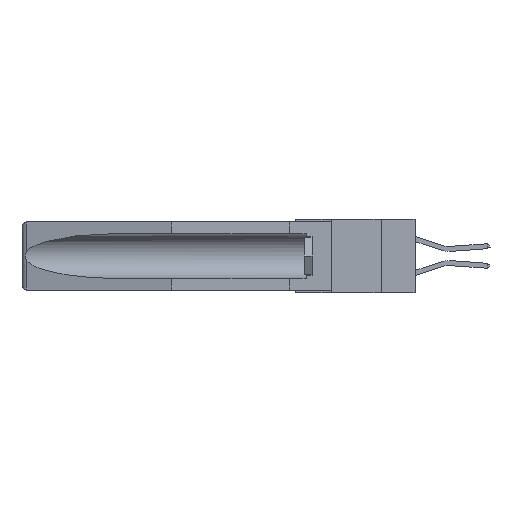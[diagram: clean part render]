
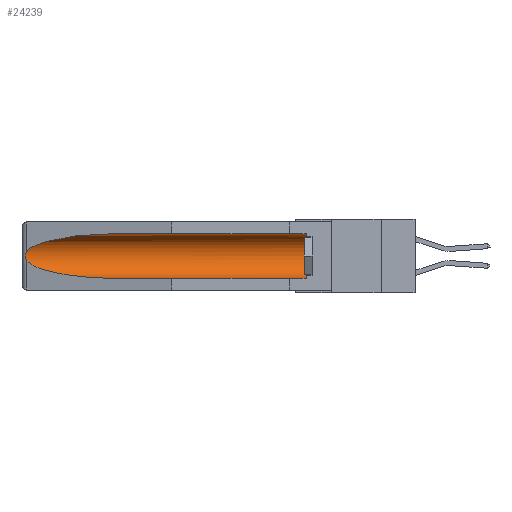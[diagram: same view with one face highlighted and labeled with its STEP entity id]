
A CAD part, left-side view. The second image highlights one B-rep face of the part: STEP entity #24239.
In plain terms, the highlighted cylindrical face has radius 2.857 mm (diameter 5.715 mm), a partial arc.
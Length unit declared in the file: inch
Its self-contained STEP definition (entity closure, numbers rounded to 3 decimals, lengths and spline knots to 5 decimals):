
#171 = CARTESIAN_POINT ( 'NONE',  ( 0.155, 1.07973, -0.284 ) ) ;
#558 = CARTESIAN_POINT ( 'NONE',  ( 0.25451, 1.48313, -0.09465 ) ) ;
#1365 = CARTESIAN_POINT ( 'NONE',  ( 0.26537, 1.52718, -0.19328 ) ) ;
#1795 = B_SPLINE_CURVE_WITH_KNOTS ( 'NONE', 3,
 ( #27884, #16819, #12589, #3488, #19022, #5691, #16997, #21360, #25749, #8009 ),
 .UNSPECIFIED., .F., .F.,
 ( 4, 2, 2, 2, 4 ),
 ( 0., 0.00029, 0.00058, 0.00087, 0.00117 ),
 .UNSPECIFIED. ) ;
#1805 = VERTEX_POINT ( 'NONE', #1365 ) ;
#3039 = EDGE_CURVE ( 'NONE', #3858, #21235, #5932, .T. ) ;
#3051 =( BOUNDED_CURVE ( )  B_SPLINE_CURVE ( 3, ( #9371, #20588, #558, #18332 ),
 .UNSPECIFIED., .F., .F. ) 
 B_SPLINE_CURVE_WITH_KNOTS ( ( 4, 4 ),
 ( 4.71239, 6.08839 ),
 .UNSPECIFIED. ) 
 CURVE ( )  GEOMETRIC_REPRESENTATION_ITEM ( )  RATIONAL_B_SPLINE_CURVE ( ( 1., 0.848, 0.848, 1. ) ) 
 REPRESENTATION_ITEM ( '' )  );
#3488 = CARTESIAN_POINT ( 'NONE',  ( 0.2673, 1.5327, -0.16383 ) ) ;
#3831 = VERTEX_POINT ( 'NONE', #23827 ) ;
#3858 = VERTEX_POINT ( 'NONE', #28498 ) ;
#5331 = DIRECTION ( 'NONE',  ( 0., 1., 0. ) ) ;
#5691 = CARTESIAN_POINT ( 'NONE',  ( 0.2675, 1.53308, -0.17534 ) ) ;
#5852 = VECTOR ( 'NONE', #23564, 39.37008 ) ;
#5932 = CIRCLE ( 'NONE', #6307, 0.1125 ) ;
#6307 = AXIS2_PLACEMENT_3D ( 'NONE', #20784, #16509, #18625 ) ;
#7411 = DIRECTION ( 'NONE',  ( 0., 1., 0. ) ) ;
#7586 = VECTOR ( 'NONE', #7411, 39.37008 ) ;
#8009 = CARTESIAN_POINT ( 'NONE',  ( 0.26537, 1.52718, -0.19328 ) ) ;
#8056 = CARTESIAN_POINT ( 'NONE',  ( 0.26537, 1.52718, -0.19328 ) ) ;
#8561 = ORIENTED_EDGE ( 'NONE', *, *, #3039, .T. ) ;
#9371 = CARTESIAN_POINT ( 'NONE',  ( 0.155, 1.07973, -0.059 ) ) ;
#9714 = LINE ( 'NONE', #23178, #5852 ) ;
#10353 = VERTEX_POINT ( 'NONE', #27807 ) ;
#11730 = CARTESIAN_POINT ( 'NONE',  ( 0.155, 0.126, -0.059 ) ) ;
#12170 = CARTESIAN_POINT ( 'NONE',  ( 0.155, -0.30754, -0.284 ) ) ;
#12542 = CARTESIAN_POINT ( 'NONE',  ( 0.21114, 1.30732, -0.284 ) ) ;
#12589 = CARTESIAN_POINT ( 'NONE',  ( 0.26654, 1.53092, -0.15636 ) ) ;
#13919 = AXIS2_PLACEMENT_3D ( 'NONE', #16935, #5331, #20921 ) ;
#14865 = EDGE_LOOP ( 'NONE', ( #19774, #23421, #25282, #19618, #8561, #22807 ) ) ;
#15461 = EDGE_CURVE ( 'NONE', #3831, #10353, #3051, .T. ) ;
#16509 = DIRECTION ( 'NONE',  ( 0., -1., 0. ) ) ;
#16819 = CARTESIAN_POINT ( 'NONE',  ( 0.26597, 1.52961, -0.15275 ) ) ;
#16935 = CARTESIAN_POINT ( 'NONE',  ( 0.155, -0.30754, -0.1715 ) ) ;
#16997 = CARTESIAN_POINT ( 'NONE',  ( 0.2673, 1.53269, -0.17917 ) ) ;
#17577 = EDGE_CURVE ( 'NONE', #21235, #3831, #9714, .T. ) ;
#17717 = LINE ( 'NONE', #12170, #7586 ) ;
#18332 = CARTESIAN_POINT ( 'NONE',  ( 0.26537, 1.52718, -0.14972 ) ) ;
#18411 = CYLINDRICAL_SURFACE ( 'NONE', #13919, 0.1125 ) ;
#18625 = DIRECTION ( 'NONE',  ( 0., 0., 1. ) ) ;
#19022 = CARTESIAN_POINT ( 'NONE',  ( 0.2675, 1.53308, -0.16763 ) ) ;
#19618 = ORIENTED_EDGE ( 'NONE', *, *, #24105, .F. ) ;
#19774 = ORIENTED_EDGE ( 'NONE', *, *, #15461, .T. ) ;
#20530 = FACE_OUTER_BOUND ( 'NONE', #14865, .T. ) ;
#20588 = CARTESIAN_POINT ( 'NONE',  ( 0.21114, 1.30732, -0.059 ) ) ;
#20697 =( BOUNDED_CURVE ( )  B_SPLINE_CURVE ( 3, ( #8056, #23745, #12542, #25971 ),
 .UNSPECIFIED., .F., .F. ) 
 B_SPLINE_CURVE_WITH_KNOTS ( ( 4, 4 ),
 ( 0.1948, 1.5708 ),
 .UNSPECIFIED. ) 
 CURVE ( )  GEOMETRIC_REPRESENTATION_ITEM ( )  RATIONAL_B_SPLINE_CURVE ( ( 1., 0.848, 0.848, 1. ) ) 
 REPRESENTATION_ITEM ( '' )  );
#20784 = CARTESIAN_POINT ( 'NONE',  ( 0.155, 0.126, -0.1715 ) ) ;
#20921 = DIRECTION ( 'NONE',  ( 0., 0., 1. ) ) ;
#21235 = VERTEX_POINT ( 'NONE', #11730 ) ;
#21360 = CARTESIAN_POINT ( 'NONE',  ( 0.26655, 1.53094, -0.18657 ) ) ;
#22551 = EDGE_CURVE ( 'NONE', #10353, #1805, #1795, .T. ) ;
#22807 = ORIENTED_EDGE ( 'NONE', *, *, #17577, .T. ) ;
#23178 = CARTESIAN_POINT ( 'NONE',  ( 0.155, -0.30754, -0.059 ) ) ;
#23378 = VERTEX_POINT ( 'NONE', #171 ) ;
#23421 = ORIENTED_EDGE ( 'NONE', *, *, #22551, .T. ) ;
#23564 = DIRECTION ( 'NONE',  ( 0., 1., 0. ) ) ;
#23745 = CARTESIAN_POINT ( 'NONE',  ( 0.25451, 1.48313, -0.24835 ) ) ;
#23827 = CARTESIAN_POINT ( 'NONE',  ( 0.155, 1.07973, -0.059 ) ) ;
#24105 = EDGE_CURVE ( 'NONE', #3858, #23378, #17717, .T. ) ;
#24239 = ADVANCED_FACE ( 'NONE', ( #20530 ), #18411, .F. ) ;
#25282 = ORIENTED_EDGE ( 'NONE', *, *, #25955, .T. ) ;
#25749 = CARTESIAN_POINT ( 'NONE',  ( 0.26597, 1.5296, -0.19026 ) ) ;
#25955 = EDGE_CURVE ( 'NONE', #1805, #23378, #20697, .T. ) ;
#25971 = CARTESIAN_POINT ( 'NONE',  ( 0.155, 1.07973, -0.284 ) ) ;
#27807 = CARTESIAN_POINT ( 'NONE',  ( 0.26537, 1.52718, -0.14972 ) ) ;
#27884 = CARTESIAN_POINT ( 'NONE',  ( 0.26537, 1.52718, -0.14972 ) ) ;
#28498 = CARTESIAN_POINT ( 'NONE',  ( 0.155, 0.126, -0.284 ) ) ;
